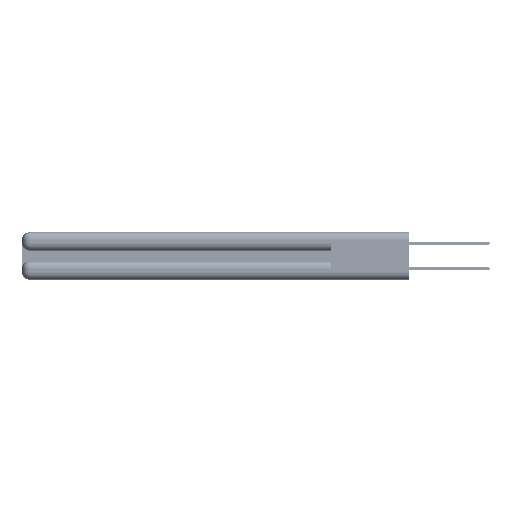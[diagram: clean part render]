
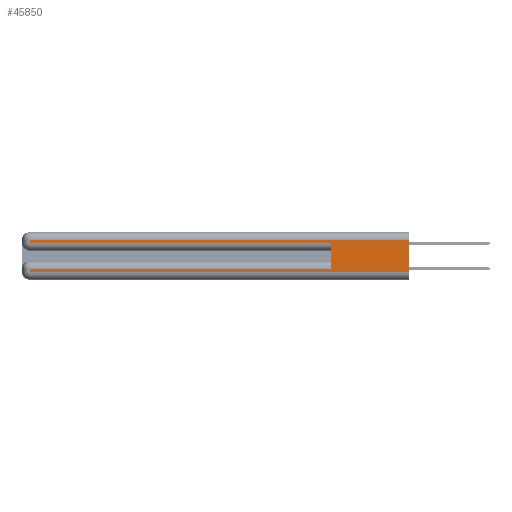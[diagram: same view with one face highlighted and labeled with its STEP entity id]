
A CAD part, left-side view. The second image highlights one B-rep face of the part: STEP entity #45850.
In plain terms, the highlighted planar face has unit normal (-1, 0, 0).
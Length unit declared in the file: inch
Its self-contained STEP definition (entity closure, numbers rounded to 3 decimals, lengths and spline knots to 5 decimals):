
#179 = DIRECTION ( 'NONE',  ( 1., 0., 0. ) ) ;
#259 = VERTEX_POINT ( 'NONE', #22649 ) ;
#1608 = CARTESIAN_POINT ( 'NONE',  ( 0., 0., 0.285 ) ) ;
#2038 = AXIS2_PLACEMENT_3D ( 'NONE', #16489, #179, #28629 ) ;
#3021 = EDGE_CURVE ( 'NONE', #3378, #52070, #37253, .T. ) ;
#3378 = VERTEX_POINT ( 'NONE', #6621 ) ;
#4144 = DIRECTION ( 'NONE',  ( 0., -1., 0. ) ) ;
#4320 = VECTOR ( 'NONE', #12707, 39.37008 ) ;
#4534 = ORIENTED_EDGE ( 'NONE', *, *, #46379, .F. ) ;
#4774 = CARTESIAN_POINT ( 'NONE',  ( 0., 2.94, 0.285 ) ) ;
#5450 = VECTOR ( 'NONE', #22974, 39.37008 ) ;
#5581 = VERTEX_POINT ( 'NONE', #4774 ) ;
#6003 = VECTOR ( 'NONE', #33904, 39.37008 ) ;
#6491 = ORIENTED_EDGE ( 'NONE', *, *, #19211, .T. ) ;
#6551 = VERTEX_POINT ( 'NONE', #11572 ) ;
#6621 = CARTESIAN_POINT ( 'NONE',  ( 0., 2.94, 0.06 ) ) ;
#7990 = VERTEX_POINT ( 'NONE', #43366 ) ;
#8176 = VECTOR ( 'NONE', #51238, 39.37008 ) ;
#9686 = CARTESIAN_POINT ( 'NONE',  ( 0., 0.6, 0.085 ) ) ;
#9739 = ORIENTED_EDGE ( 'NONE', *, *, #44265, .T. ) ;
#9889 = DIRECTION ( 'NONE',  ( 0., -1., 0. ) ) ;
#11572 = CARTESIAN_POINT ( 'NONE',  ( 0., 0., 0.31 ) ) ;
#11739 = CARTESIAN_POINT ( 'NONE',  ( 0., 0., 0.085 ) ) ;
#11940 = VECTOR ( 'NONE', #9889, 39.37008 ) ;
#12707 = DIRECTION ( 'NONE',  ( 0., 0., -1. ) ) ;
#14991 = EDGE_CURVE ( 'NONE', #5581, #7990, #33423, .T. ) ;
#15147 = EDGE_CURVE ( 'NONE', #259, #3378, #29619, .T. ) ;
#15617 = VECTOR ( 'NONE', #15823, 39.37008 ) ;
#15823 = DIRECTION ( 'NONE',  ( 0., 1., 0. ) ) ;
#16489 = CARTESIAN_POINT ( 'NONE',  ( 0., 0., 0.37 ) ) ;
#17399 = ORIENTED_EDGE ( 'NONE', *, *, #15147, .T. ) ;
#18907 = CARTESIAN_POINT ( 'NONE',  ( 0., 2.94, 0.37 ) ) ;
#19211 = EDGE_CURVE ( 'NONE', #49658, #259, #37099, .T. ) ;
#19248 = ORIENTED_EDGE ( 'NONE', *, *, #39717, .T. ) ;
#20568 = CARTESIAN_POINT ( 'NONE',  ( 0., 0., 0.06 ) ) ;
#21181 = ORIENTED_EDGE ( 'NONE', *, *, #3021, .T. ) ;
#22649 = CARTESIAN_POINT ( 'NONE',  ( 0., 2.94, 0.085 ) ) ;
#22974 = DIRECTION ( 'NONE',  ( 0., 0., -1. ) ) ;
#27091 = CARTESIAN_POINT ( 'NONE',  ( 0., 0., 0.31 ) ) ;
#27225 = LINE ( 'NONE', #27091, #8176 ) ;
#28629 = DIRECTION ( 'NONE',  ( 0., 0., -1. ) ) ;
#29619 = LINE ( 'NONE', #18907, #5450 ) ;
#29837 = CARTESIAN_POINT ( 'NONE',  ( 0., 0.6, 0.145 ) ) ;
#31134 = CARTESIAN_POINT ( 'NONE',  ( 0., 2.94, 0.31 ) ) ;
#32504 = EDGE_LOOP ( 'NONE', ( #4534, #19248, #9739, #44498, #35081, #6491, #17399, #21181 ) ) ;
#33423 = LINE ( 'NONE', #1608, #11940 ) ;
#33783 = VERTEX_POINT ( 'NONE', #31134 ) ;
#33904 = DIRECTION ( 'NONE',  ( 0., 0., 1. ) ) ;
#34449 = LINE ( 'NONE', #46794, #52081 ) ;
#35081 = ORIENTED_EDGE ( 'NONE', *, *, #49656, .F. ) ;
#35494 = LINE ( 'NONE', #36929, #4320 ) ;
#36929 = CARTESIAN_POINT ( 'NONE',  ( 0., 0., 0.37 ) ) ;
#37099 = LINE ( 'NONE', #11739, #15617 ) ;
#37253 = LINE ( 'NONE', #20568, #47927 ) ;
#38398 = LINE ( 'NONE', #29837, #6003 ) ;
#39314 = FACE_OUTER_BOUND ( 'NONE', #32504, .T. ) ;
#39717 = EDGE_CURVE ( 'NONE', #6551, #33783, #27225, .T. ) ;
#40932 = CARTESIAN_POINT ( 'NONE',  ( 0., 0., 0.06 ) ) ;
#43366 = CARTESIAN_POINT ( 'NONE',  ( 0., 0.6, 0.285 ) ) ;
#44265 = EDGE_CURVE ( 'NONE', #33783, #5581, #34449, .T. ) ;
#44498 = ORIENTED_EDGE ( 'NONE', *, *, #14991, .T. ) ;
#45850 = ADVANCED_FACE ( 'NONE', ( #39314 ), #48737, .F. ) ;
#46379 = EDGE_CURVE ( 'NONE', #6551, #52070, #35494, .T. ) ;
#46794 = CARTESIAN_POINT ( 'NONE',  ( 0., 2.94, 0.37 ) ) ;
#47927 = VECTOR ( 'NONE', #4144, 39.37008 ) ;
#48737 = PLANE ( 'NONE',  #2038 ) ;
#49656 = EDGE_CURVE ( 'NONE', #49658, #7990, #38398, .T. ) ;
#49658 = VERTEX_POINT ( 'NONE', #9686 ) ;
#50838 = DIRECTION ( 'NONE',  ( 0., 0., -1. ) ) ;
#51238 = DIRECTION ( 'NONE',  ( 0., 1., 0. ) ) ;
#52070 = VERTEX_POINT ( 'NONE', #40932 ) ;
#52081 = VECTOR ( 'NONE', #50838, 39.37008 ) ;
